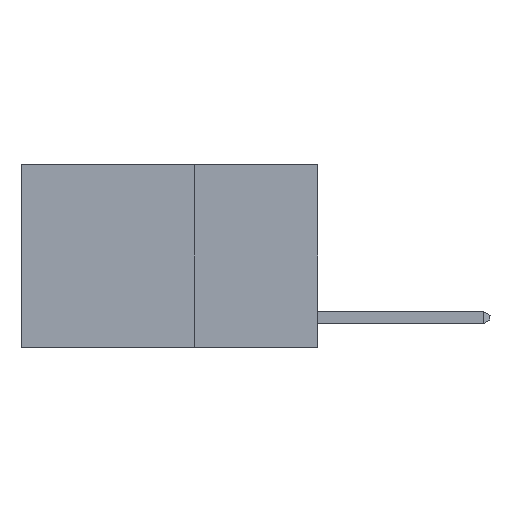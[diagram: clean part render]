
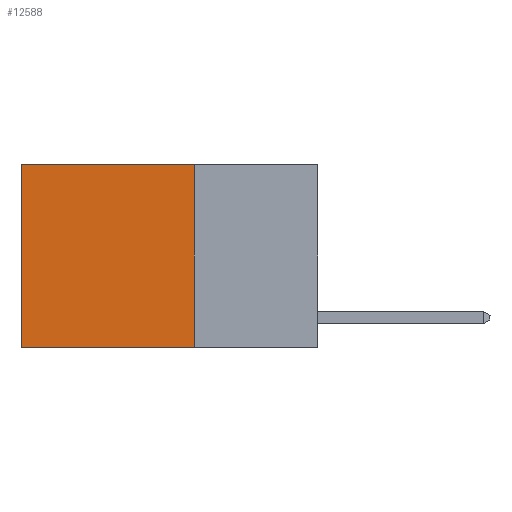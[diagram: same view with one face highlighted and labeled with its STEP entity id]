
A CAD part, left-side view. The second image highlights one B-rep face of the part: STEP entity #12588.
In plain terms, the highlighted planar face has unit normal (-1, 0, 0).
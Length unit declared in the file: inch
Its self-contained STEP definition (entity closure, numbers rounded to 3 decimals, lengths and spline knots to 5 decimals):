
#79 = EDGE_LOOP ( 'NONE', ( #12593, #14021, #20565, #7799 ) ) ;
#516 = CARTESIAN_POINT ( 'NONE',  ( 0.2625, 0.6, 0. ) ) ;
#1181 = PLANE ( 'NONE',  #20062 ) ;
#2255 = VECTOR ( 'NONE', #16870, 39.37008 ) ;
#2765 = EDGE_CURVE ( 'NONE', #10222, #17957, #17561, .T. ) ;
#5063 = VECTOR ( 'NONE', #19063, 39.37008 ) ;
#5319 = CARTESIAN_POINT ( 'NONE',  ( 0.2625, 0.25, 0. ) ) ;
#6154 = EDGE_CURVE ( 'NONE', #18460, #8138, #7223, .T. ) ;
#6719 = FACE_OUTER_BOUND ( 'NONE', #79, .T. ) ;
#7223 = LINE ( 'NONE', #5319, #2255 ) ;
#7228 = DIRECTION ( 'NONE',  ( 0., 0., -1. ) ) ;
#7637 = LINE ( 'NONE', #9743, #20049 ) ;
#7799 = ORIENTED_EDGE ( 'NONE', *, *, #17134, .T. ) ;
#8138 = VERTEX_POINT ( 'NONE', #9634 ) ;
#9570 = CARTESIAN_POINT ( 'NONE',  ( 0.2625, 0.25, 0. ) ) ;
#9634 = CARTESIAN_POINT ( 'NONE',  ( 0.2625, 0.25, -0.37 ) ) ;
#9743 = CARTESIAN_POINT ( 'NONE',  ( 0.2625, 0.25, 0. ) ) ;
#9974 = CARTESIAN_POINT ( 'NONE',  ( 0.2625, 0.6, 0. ) ) ;
#10222 = VERTEX_POINT ( 'NONE', #9974 ) ;
#11233 = DIRECTION ( 'NONE',  ( 0., 0., -1. ) ) ;
#11726 = CARTESIAN_POINT ( 'NONE',  ( 0.2625, 0.25, 0. ) ) ;
#12588 = ADVANCED_FACE ( 'NONE', ( #6719 ), #1181, .F. ) ;
#12593 = ORIENTED_EDGE ( 'NONE', *, *, #2765, .T. ) ;
#14021 = ORIENTED_EDGE ( 'NONE', *, *, #16008, .F. ) ;
#14328 = CARTESIAN_POINT ( 'NONE',  ( 0.2625, 0.25, -0.37 ) ) ;
#16008 = EDGE_CURVE ( 'NONE', #8138, #17957, #18132, .T. ) ;
#16289 = DIRECTION ( 'NONE',  ( 0., 1., 0. ) ) ;
#16870 = DIRECTION ( 'NONE',  ( 0., 0., -1. ) ) ;
#17134 = EDGE_CURVE ( 'NONE', #18460, #10222, #7637, .T. ) ;
#17561 = LINE ( 'NONE', #516, #20796 ) ;
#17957 = VERTEX_POINT ( 'NONE', #18297 ) ;
#18132 = LINE ( 'NONE', #14328, #5063 ) ;
#18297 = CARTESIAN_POINT ( 'NONE',  ( 0.2625, 0.6, -0.37 ) ) ;
#18460 = VERTEX_POINT ( 'NONE', #11726 ) ;
#19063 = DIRECTION ( 'NONE',  ( 0., 1., 0. ) ) ;
#20049 = VECTOR ( 'NONE', #16289, 39.37008 ) ;
#20062 = AXIS2_PLACEMENT_3D ( 'NONE', #9570, #20850, #11233 ) ;
#20565 = ORIENTED_EDGE ( 'NONE', *, *, #6154, .F. ) ;
#20796 = VECTOR ( 'NONE', #7228, 39.37008 ) ;
#20850 = DIRECTION ( 'NONE',  ( 1., 0., 0. ) ) ;
